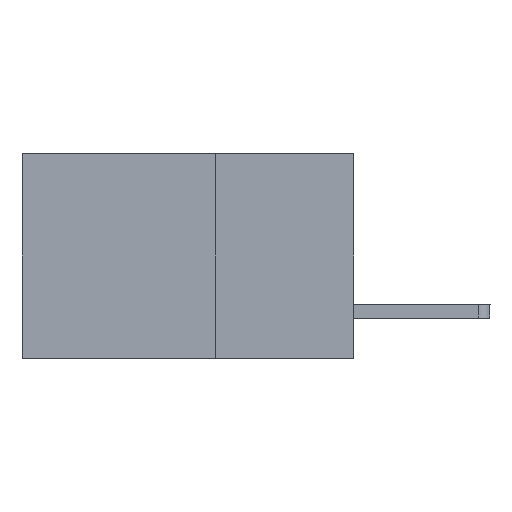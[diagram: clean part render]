
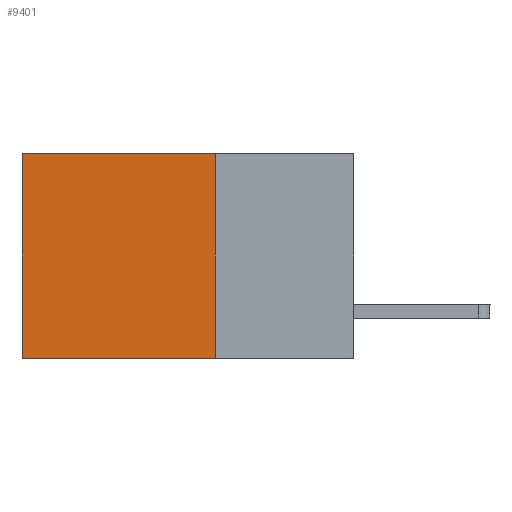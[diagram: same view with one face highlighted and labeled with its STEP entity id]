
A CAD part, left-side view. The second image highlights one B-rep face of the part: STEP entity #9401.
In plain terms, the highlighted planar face has unit normal (-1, 0, 0).
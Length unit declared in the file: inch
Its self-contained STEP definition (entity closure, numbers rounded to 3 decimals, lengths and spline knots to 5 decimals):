
#15 = LINE ( 'NONE', #8157, #9822 ) ;
#200 = CARTESIAN_POINT ( 'NONE',  ( 0.2875, 0.6, 0. ) ) ;
#504 = ORIENTED_EDGE ( 'NONE', *, *, #11476, .F. ) ;
#524 = ORIENTED_EDGE ( 'NONE', *, *, #7063, .T. ) ;
#880 = VECTOR ( 'NONE', #2853, 39.37008 ) ;
#1318 = VERTEX_POINT ( 'NONE', #6622 ) ;
#1528 = ORIENTED_EDGE ( 'NONE', *, *, #7137, .F. ) ;
#1586 = CARTESIAN_POINT ( 'NONE',  ( 0.2875, 0.25, 0. ) ) ;
#2084 = VECTOR ( 'NONE', #3999, 39.37008 ) ;
#2674 = AXIS2_PLACEMENT_3D ( 'NONE', #1586, #3550, #9783 ) ;
#2853 = DIRECTION ( 'NONE',  ( 0., 1., 0. ) ) ;
#2994 = VERTEX_POINT ( 'NONE', #5437 ) ;
#3550 = DIRECTION ( 'NONE',  ( 1., 0., 0. ) ) ;
#3999 = DIRECTION ( 'NONE',  ( 0., 0., -1. ) ) ;
#4162 = EDGE_LOOP ( 'NONE', ( #4859, #1528, #504, #524 ) ) ;
#4344 = DIRECTION ( 'NONE',  ( 0., 0., -1. ) ) ;
#4520 = LINE ( 'NONE', #200, #2084 ) ;
#4551 = CARTESIAN_POINT ( 'NONE',  ( 0.2875, 0.6, -0.37 ) ) ;
#4580 = CARTESIAN_POINT ( 'NONE',  ( 0.2875, 0.25, -0.37 ) ) ;
#4700 = DIRECTION ( 'NONE',  ( 0., 1., 0. ) ) ;
#4859 = ORIENTED_EDGE ( 'NONE', *, *, #10338, .T. ) ;
#5437 = CARTESIAN_POINT ( 'NONE',  ( 0.2875, 0.25, 0. ) ) ;
#6008 = PLANE ( 'NONE',  #2674 ) ;
#6622 = CARTESIAN_POINT ( 'NONE',  ( 0.2875, 0.6, 0. ) ) ;
#6648 = FACE_OUTER_BOUND ( 'NONE', #4162, .T. ) ;
#7017 = VERTEX_POINT ( 'NONE', #4551 ) ;
#7063 = EDGE_CURVE ( 'NONE', #2994, #1318, #15, .T. ) ;
#7137 = EDGE_CURVE ( 'NONE', #10565, #7017, #9849, .T. ) ;
#8157 = CARTESIAN_POINT ( 'NONE',  ( 0.2875, 0.25, 0. ) ) ;
#8164 = CARTESIAN_POINT ( 'NONE',  ( 0.2875, 0.25, -0.37 ) ) ;
#9401 = ADVANCED_FACE ( 'NONE', ( #6648 ), #6008, .F. ) ;
#9783 = DIRECTION ( 'NONE',  ( 0., 0., -1. ) ) ;
#9822 = VECTOR ( 'NONE', #4700, 39.37008 ) ;
#9845 = CARTESIAN_POINT ( 'NONE',  ( 0.2875, 0.25, 0. ) ) ;
#9849 = LINE ( 'NONE', #4580, #880 ) ;
#10176 = VECTOR ( 'NONE', #4344, 39.37008 ) ;
#10338 = EDGE_CURVE ( 'NONE', #1318, #7017, #4520, .T. ) ;
#10465 = LINE ( 'NONE', #9845, #10176 ) ;
#10565 = VERTEX_POINT ( 'NONE', #8164 ) ;
#11476 = EDGE_CURVE ( 'NONE', #2994, #10565, #10465, .T. ) ;
